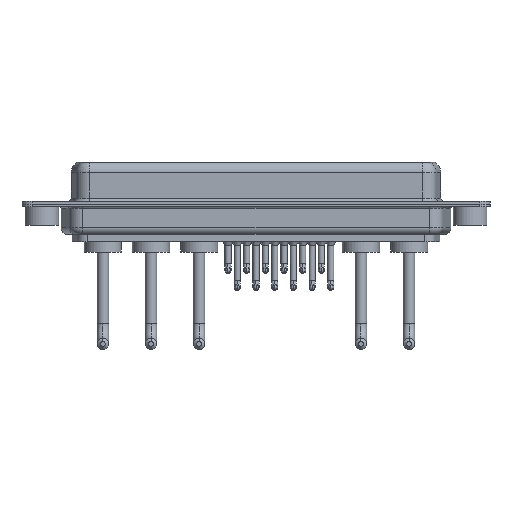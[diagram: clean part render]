
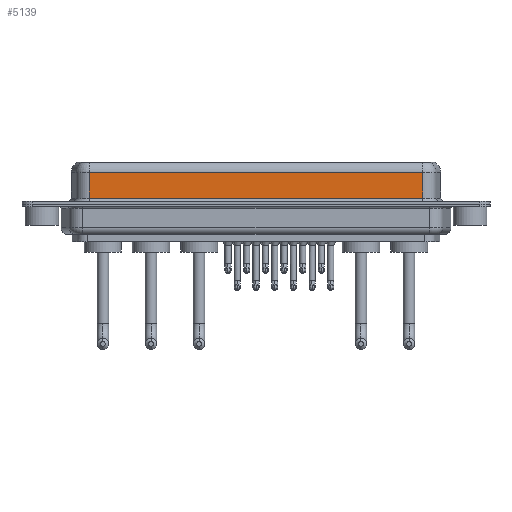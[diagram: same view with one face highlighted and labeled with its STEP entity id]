
A CAD part, front view. The second image highlights one B-rep face of the part: STEP entity #5139.
In plain terms, the highlighted planar face has unit normal (0, -1, 0).
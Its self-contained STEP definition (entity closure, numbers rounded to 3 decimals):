
#1438 = ORIENTED_EDGE ( 'NONE', *, *, #16021, .T. ) ;
#1620 = EDGE_CURVE ( 'NONE', #8439, #6572, #12230, .T. ) ;
#2515 = EDGE_LOOP ( 'NONE', ( #5461, #1438, #2581, #6325 ) ) ;
#2581 = ORIENTED_EDGE ( 'NONE', *, *, #1620, .T. ) ;
#2923 = VECTOR ( 'NONE', #13582, 1000. ) ;
#4099 = DIRECTION ( 'NONE',  ( -1., 0., 0. ) ) ;
#4404 = VECTOR ( 'NONE', #5366, 1000. ) ;
#4455 = VERTEX_POINT ( 'NONE', #7762 ) ;
#5139 = ADVANCED_FACE ( 'NONE', ( #15690 ), #9344, .F. ) ;
#5366 = DIRECTION ( 'NONE',  ( 1., 0., 0. ) ) ;
#5461 = ORIENTED_EDGE ( 'NONE', *, *, #13518, .F. ) ;
#5579 = VECTOR ( 'NONE', #4099, 1000. ) ;
#5646 = CARTESIAN_POINT ( 'NONE',  ( 56.462, -3.95, 4.65 ) ) ;
#5756 = VECTOR ( 'NONE', #15305, 1000. ) ;
#6325 = ORIENTED_EDGE ( 'NONE', *, *, #20079, .T. ) ;
#6572 = VERTEX_POINT ( 'NONE', #10141 ) ;
#7762 = CARTESIAN_POINT ( 'NONE',  ( 56.462, -3.95, 0.9 ) ) ;
#7915 = DIRECTION ( 'NONE',  ( 0., 0., 1. ) ) ;
#8439 = VERTEX_POINT ( 'NONE', #13793 ) ;
#8695 = LINE ( 'NONE', #5646, #5579 ) ;
#9344 = PLANE ( 'NONE',  #13753 ) ;
#10141 = CARTESIAN_POINT ( 'NONE',  ( 7.038, -3.95, 0.9 ) ) ;
#11391 = VERTEX_POINT ( 'NONE', #17116 ) ;
#12230 = LINE ( 'NONE', #15096, #5756 ) ;
#12400 = DIRECTION ( 'NONE',  ( 0., 1., 0. ) ) ;
#13518 = EDGE_CURVE ( 'NONE', #11391, #4455, #16480, .T. ) ;
#13582 = DIRECTION ( 'NONE',  ( 0., 0., -1. ) ) ;
#13753 = AXIS2_PLACEMENT_3D ( 'NONE', #18655, #12400, #7915 ) ;
#13787 = CARTESIAN_POINT ( 'NONE',  ( 56.462, -3.95, 6.4 ) ) ;
#13793 = CARTESIAN_POINT ( 'NONE',  ( 7.038, -3.95, 4.65 ) ) ;
#15096 = CARTESIAN_POINT ( 'NONE',  ( 7.038, -3.95, 6.4 ) ) ;
#15305 = DIRECTION ( 'NONE',  ( 0., 0., -1. ) ) ;
#15690 = FACE_OUTER_BOUND ( 'NONE', #2515, .T. ) ;
#16021 = EDGE_CURVE ( 'NONE', #11391, #8439, #8695, .T. ) ;
#16480 = LINE ( 'NONE', #13787, #2923 ) ;
#17116 = CARTESIAN_POINT ( 'NONE',  ( 56.462, -3.95, 4.65 ) ) ;
#17945 = LINE ( 'NONE', #19377, #4404 ) ;
#18655 = CARTESIAN_POINT ( 'NONE',  ( 56.462, -3.95, 6.4 ) ) ;
#19377 = CARTESIAN_POINT ( 'NONE',  ( 56.462, -3.95, 0.9 ) ) ;
#20079 = EDGE_CURVE ( 'NONE', #6572, #4455, #17945, .T. ) ;
